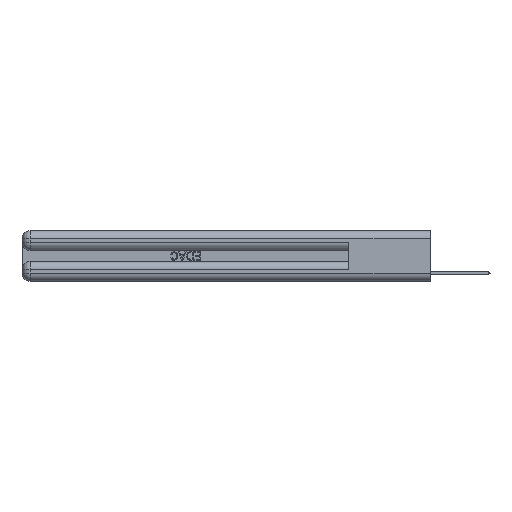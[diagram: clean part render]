
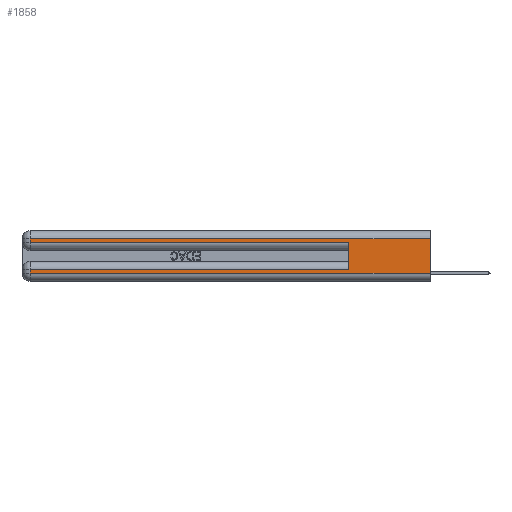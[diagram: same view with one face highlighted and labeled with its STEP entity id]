
A CAD part, left-side view. The second image highlights one B-rep face of the part: STEP entity #1858.
In plain terms, the highlighted planar face has unit normal (-1, 0, 0).
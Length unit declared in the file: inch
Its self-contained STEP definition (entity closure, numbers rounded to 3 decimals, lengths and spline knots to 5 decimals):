
#1546 = EDGE_CURVE ( 'NONE', #1826, #1775, #25157, .T. ) ;
#1775 = VERTEX_POINT ( 'NONE', #5140 ) ;
#1826 = VERTEX_POINT ( 'NONE', #18935 ) ;
#1858 = ADVANCED_FACE ( 'NONE', ( #4124 ), #22872, .F. ) ;
#2121 = CARTESIAN_POINT ( 'NONE',  ( 0., 0., 0.06 ) ) ;
#2271 = AXIS2_PLACEMENT_3D ( 'NONE', #3983, #21035, #5964 ) ;
#2555 = CARTESIAN_POINT ( 'NONE',  ( 0., 0., 0.285 ) ) ;
#3336 = CARTESIAN_POINT ( 'NONE',  ( 0., 2.94, 0.37 ) ) ;
#3459 = EDGE_CURVE ( 'NONE', #22115, #22028, #27341, .T. ) ;
#3983 = CARTESIAN_POINT ( 'NONE',  ( 0., 0., 0.37 ) ) ;
#4102 = VECTOR ( 'NONE', #14254, 39.37008 ) ;
#4124 = FACE_OUTER_BOUND ( 'NONE', #19272, .T. ) ;
#4232 = EDGE_CURVE ( 'NONE', #22115, #24238, #14147, .T. ) ;
#4659 = EDGE_CURVE ( 'NONE', #24238, #27130, #17817, .T. ) ;
#4682 = ORIENTED_EDGE ( 'NONE', *, *, #25992, .T. ) ;
#5103 = DIRECTION ( 'NONE',  ( 0., -1., 0. ) ) ;
#5140 = CARTESIAN_POINT ( 'NONE',  ( 0., 2.94, 0.31 ) ) ;
#5277 = VECTOR ( 'NONE', #5103, 39.37008 ) ;
#5292 = CARTESIAN_POINT ( 'NONE',  ( 0., 0., 0.085 ) ) ;
#5684 = CARTESIAN_POINT ( 'NONE',  ( 0., 0., 0.37 ) ) ;
#5860 = DIRECTION ( 'NONE',  ( 0., 1., 0. ) ) ;
#5964 = DIRECTION ( 'NONE',  ( 0., 0., -1. ) ) ;
#6372 = DIRECTION ( 'NONE',  ( 0., -1., 0. ) ) ;
#7264 = ORIENTED_EDGE ( 'NONE', *, *, #10216, .F. ) ;
#9245 = CARTESIAN_POINT ( 'NONE',  ( 0., 0.6, 0.085 ) ) ;
#9936 = DIRECTION ( 'NONE',  ( 0., 1., 0. ) ) ;
#10040 = CARTESIAN_POINT ( 'NONE',  ( 0., 0.6, 0.145 ) ) ;
#10216 = EDGE_CURVE ( 'NONE', #1826, #23415, #21030, .T. ) ;
#10498 = EDGE_CURVE ( 'NONE', #19107, #22028, #24260, .T. ) ;
#10627 = CARTESIAN_POINT ( 'NONE',  ( 0., 0., 0.06 ) ) ;
#11175 = DIRECTION ( 'NONE',  ( 0., 0., -1. ) ) ;
#11697 = CARTESIAN_POINT ( 'NONE',  ( 0., 2.94, 0.285 ) ) ;
#12427 = VECTOR ( 'NONE', #11175, 39.37008 ) ;
#12432 = ORIENTED_EDGE ( 'NONE', *, *, #1546, .T. ) ;
#12730 = ORIENTED_EDGE ( 'NONE', *, *, #3459, .F. ) ;
#14147 = LINE ( 'NONE', #5292, #21122 ) ;
#14254 = DIRECTION ( 'NONE',  ( 0., 0., -1. ) ) ;
#14953 = ORIENTED_EDGE ( 'NONE', *, *, #4232, .T. ) ;
#15717 = CARTESIAN_POINT ( 'NONE',  ( 0., 2.94, 0.06 ) ) ;
#15897 = LINE ( 'NONE', #3336, #18718 ) ;
#17817 = LINE ( 'NONE', #26398, #12427 ) ;
#18718 = VECTOR ( 'NONE', #26869, 39.37008 ) ;
#18767 = DIRECTION ( 'NONE',  ( 0., 0., 1. ) ) ;
#18935 = CARTESIAN_POINT ( 'NONE',  ( 0., 0., 0.31 ) ) ;
#19107 = VERTEX_POINT ( 'NONE', #11697 ) ;
#19272 = EDGE_LOOP ( 'NONE', ( #7264, #12432, #26961, #25565, #12730, #14953, #21318, #4682 ) ) ;
#19787 = VECTOR ( 'NONE', #5860, 39.37008 ) ;
#21030 = LINE ( 'NONE', #5684, #4102 ) ;
#21035 = DIRECTION ( 'NONE',  ( 1., 0., 0. ) ) ;
#21122 = VECTOR ( 'NONE', #9936, 39.37008 ) ;
#21318 = ORIENTED_EDGE ( 'NONE', *, *, #4659, .T. ) ;
#21815 = EDGE_CURVE ( 'NONE', #1775, #19107, #15897, .T. ) ;
#22028 = VERTEX_POINT ( 'NONE', #27416 ) ;
#22115 = VERTEX_POINT ( 'NONE', #9245 ) ;
#22872 = PLANE ( 'NONE',  #2271 ) ;
#23415 = VERTEX_POINT ( 'NONE', #10627 ) ;
#24238 = VERTEX_POINT ( 'NONE', #24850 ) ;
#24260 = LINE ( 'NONE', #2555, #5277 ) ;
#24850 = CARTESIAN_POINT ( 'NONE',  ( 0., 2.94, 0.085 ) ) ;
#25016 = CARTESIAN_POINT ( 'NONE',  ( 0., 0., 0.31 ) ) ;
#25157 = LINE ( 'NONE', #25016, #19787 ) ;
#25565 = ORIENTED_EDGE ( 'NONE', *, *, #10498, .T. ) ;
#25992 = EDGE_CURVE ( 'NONE', #27130, #23415, #27626, .T. ) ;
#26398 = CARTESIAN_POINT ( 'NONE',  ( 0., 2.94, 0.37 ) ) ;
#26869 = DIRECTION ( 'NONE',  ( 0., 0., -1. ) ) ;
#26882 = VECTOR ( 'NONE', #18767, 39.37008 ) ;
#26961 = ORIENTED_EDGE ( 'NONE', *, *, #21815, .T. ) ;
#26993 = VECTOR ( 'NONE', #6372, 39.37008 ) ;
#27130 = VERTEX_POINT ( 'NONE', #15717 ) ;
#27341 = LINE ( 'NONE', #10040, #26882 ) ;
#27416 = CARTESIAN_POINT ( 'NONE',  ( 0., 0.6, 0.285 ) ) ;
#27626 = LINE ( 'NONE', #2121, #26993 ) ;
